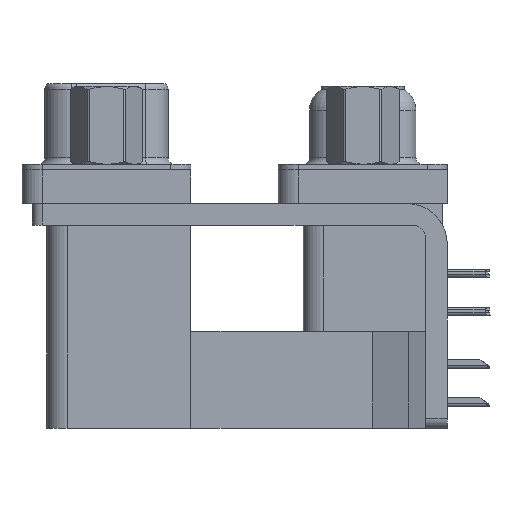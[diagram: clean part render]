
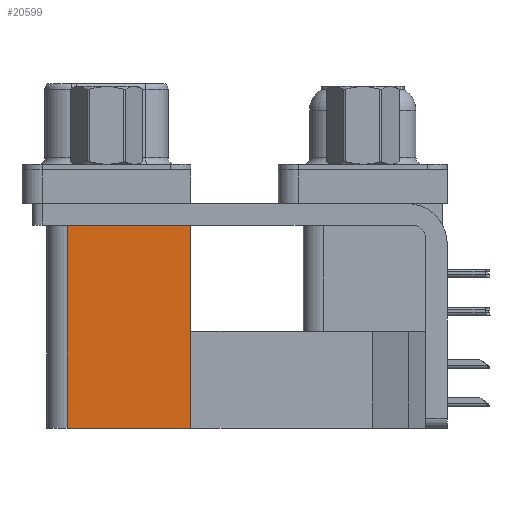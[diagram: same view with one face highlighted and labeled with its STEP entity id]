
A CAD part, left-side view. The second image highlights one B-rep face of the part: STEP entity #20599.
In plain terms, the highlighted planar face has unit normal (-1, 0, 0).
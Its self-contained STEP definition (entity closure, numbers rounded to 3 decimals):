
#215 = VECTOR ( 'NONE', #11394, 1000. ) ;
#421 = DIRECTION ( 'NONE',  ( 1., 0., 0. ) ) ;
#1027 = VERTEX_POINT ( 'NONE', #26875 ) ;
#1371 = CARTESIAN_POINT ( 'NONE',  ( 3.79, 12.775, -2.5 ) ) ;
#1833 = AXIS2_PLACEMENT_3D ( 'NONE', #29608, #421, #40613 ) ;
#2492 = EDGE_CURVE ( 'NONE', #1027, #25100, #41986, .T. ) ;
#2939 = ORIENTED_EDGE ( 'NONE', *, *, #2492, .T. ) ;
#5251 = CARTESIAN_POINT ( 'NONE',  ( 3.79, 12.775, -19.2 ) ) ;
#5828 = DIRECTION ( 'NONE',  ( 0., 0., 1. ) ) ;
#8613 = ORIENTED_EDGE ( 'NONE', *, *, #25225, .T. ) ;
#10905 = VECTOR ( 'NONE', #20971, 1000. ) ;
#11162 = LINE ( 'NONE', #24171, #10905 ) ;
#11394 = DIRECTION ( 'NONE',  ( 0., 0., 1. ) ) ;
#11677 = CARTESIAN_POINT ( 'NONE',  ( 3.79, 21.975, -2.5 ) ) ;
#13094 = VERTEX_POINT ( 'NONE', #11677 ) ;
#14818 = ORIENTED_EDGE ( 'NONE', *, *, #23470, .F. ) ;
#17110 = EDGE_LOOP ( 'NONE', ( #8613, #23834, #14818, #2939 ) ) ;
#18807 = VECTOR ( 'NONE', #5828, 1000. ) ;
#20599 = ADVANCED_FACE ( 'NONE', ( #35976 ), #32782, .F. ) ;
#20971 = DIRECTION ( 'NONE',  ( 0., 1., 0. ) ) ;
#23470 = EDGE_CURVE ( 'NONE', #1027, #41546, #35062, .T. ) ;
#23834 = ORIENTED_EDGE ( 'NONE', *, *, #40322, .F. ) ;
#24171 = CARTESIAN_POINT ( 'NONE',  ( 3.79, 12.775, -2.5 ) ) ;
#25100 = VERTEX_POINT ( 'NONE', #1371 ) ;
#25225 = EDGE_CURVE ( 'NONE', #25100, #13094, #11162, .T. ) ;
#26875 = CARTESIAN_POINT ( 'NONE',  ( 3.79, 12.775, -19.2 ) ) ;
#28446 = CARTESIAN_POINT ( 'NONE',  ( 3.79, 21.975, -19.2 ) ) ;
#29204 = VECTOR ( 'NONE', #31429, 1000. ) ;
#29608 = CARTESIAN_POINT ( 'NONE',  ( 3.79, 12.775, -19.2 ) ) ;
#31429 = DIRECTION ( 'NONE',  ( 0., 1., 0. ) ) ;
#31621 = LINE ( 'NONE', #28446, #215 ) ;
#32782 = PLANE ( 'NONE',  #1833 ) ;
#34992 = CARTESIAN_POINT ( 'NONE',  ( 3.79, 12.775, -19.2 ) ) ;
#35062 = LINE ( 'NONE', #5251, #29204 ) ;
#35976 = FACE_OUTER_BOUND ( 'NONE', #17110, .T. ) ;
#39520 = CARTESIAN_POINT ( 'NONE',  ( 3.79, 21.975, -19.2 ) ) ;
#40322 = EDGE_CURVE ( 'NONE', #41546, #13094, #31621, .T. ) ;
#40613 = DIRECTION ( 'NONE',  ( 0., 0., -1. ) ) ;
#41546 = VERTEX_POINT ( 'NONE', #39520 ) ;
#41986 = LINE ( 'NONE', #34992, #18807 ) ;
